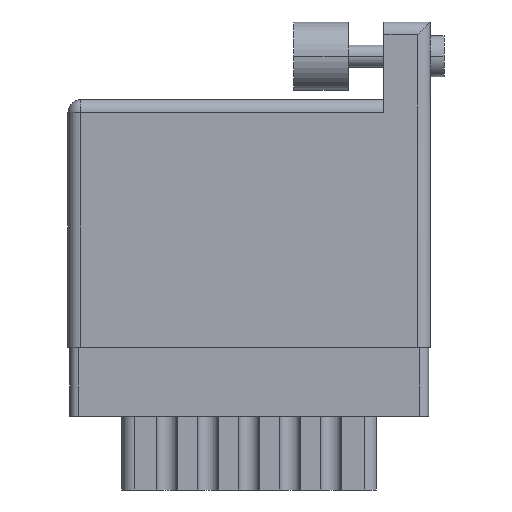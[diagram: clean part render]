
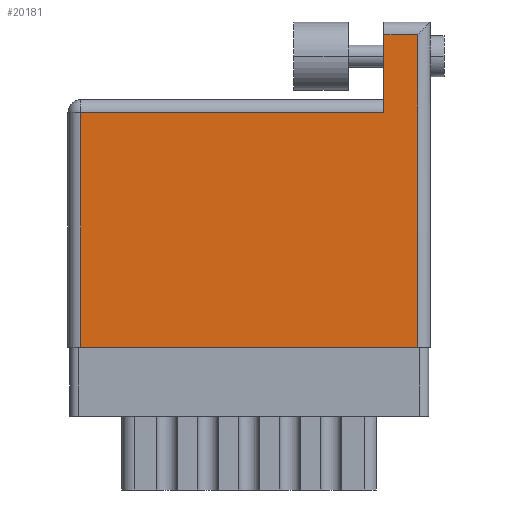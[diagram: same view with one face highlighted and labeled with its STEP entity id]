
A CAD part, front view. The second image highlights one B-rep face of the part: STEP entity #20181.
In plain terms, the highlighted face is planar.
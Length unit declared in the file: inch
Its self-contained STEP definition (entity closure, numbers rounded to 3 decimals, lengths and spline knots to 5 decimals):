
#1855 = CARTESIAN_POINT ( 'NONE',  ( 0., 0.859, 0. ) ) ;
#1906 = DIRECTION ( 'NONE',  ( 0., 1., 0. ) ) ;
#3386 = CARTESIAN_POINT ( 'NONE',  ( 1.155, 1.19, 0. ) ) ;
#3553 = VERTEX_POINT ( 'NONE', #25273 ) ;
#4104 = VERTEX_POINT ( 'NONE', #6289 ) ;
#4347 = LINE ( 'NONE', #1855, #9684 ) ;
#4431 = EDGE_CURVE ( 'NONE', #9054, #4104, #13331, .T. ) ;
#5066 = EDGE_CURVE ( 'NONE', #5283, #9054, #16066, .T. ) ;
#5283 = VERTEX_POINT ( 'NONE', #16950 ) ;
#5483 = LINE ( 'NONE', #3386, #15075 ) ;
#6289 = CARTESIAN_POINT ( 'NONE',  ( 1.155, 1.143, 0. ) ) ;
#7041 = VERTEX_POINT ( 'NONE', #9568 ) ;
#7189 = DIRECTION ( 'NONE',  ( -1., 0., 0. ) ) ;
#7658 = VECTOR ( 'NONE', #8145, 39.37008 ) ;
#7846 = ORIENTED_EDGE ( 'NONE', *, *, #21690, .T. ) ;
#7950 = CARTESIAN_POINT ( 'NONE',  ( 1.278, 1.143, 0. ) ) ;
#8145 = DIRECTION ( 'NONE',  ( 1., 0., 0. ) ) ;
#9054 = VERTEX_POINT ( 'NONE', #7950 ) ;
#9568 = CARTESIAN_POINT ( 'NONE',  ( 0.047, 0., 0. ) ) ;
#9684 = VECTOR ( 'NONE', #23977, 39.37008 ) ;
#9896 = CARTESIAN_POINT ( 'NONE',  ( 1.278, 1.19, 0. ) ) ;
#10797 = CARTESIAN_POINT ( 'NONE',  ( 0.047, 0.859, 0. ) ) ;
#11574 = LINE ( 'NONE', #21392, #7658 ) ;
#12564 = VECTOR ( 'NONE', #1906, 39.37008 ) ;
#13205 = DIRECTION ( 'NONE',  ( 0., -1., 0. ) ) ;
#13311 = DIRECTION ( 'NONE',  ( 0., 0., -1. ) ) ;
#13331 = LINE ( 'NONE', #23404, #21728 ) ;
#13974 = EDGE_LOOP ( 'NONE', ( #7846, #18714, #19465, #24093, #22214, #21532 ) ) ;
#14175 = EDGE_CURVE ( 'NONE', #4104, #3553, #5483, .T. ) ;
#15075 = VECTOR ( 'NONE', #13205, 39.37008 ) ;
#15550 = CARTESIAN_POINT ( 'NONE',  ( 0., 0.906, 0. ) ) ;
#16014 = EDGE_CURVE ( 'NONE', #22884, #7041, #19489, .T. ) ;
#16066 = LINE ( 'NONE', #9896, #12564 ) ;
#16950 = CARTESIAN_POINT ( 'NONE',  ( 1.278, 0., 0. ) ) ;
#17516 = DIRECTION ( 'NONE',  ( 0., -1., 0. ) ) ;
#17633 = AXIS2_PLACEMENT_3D ( 'NONE', #15550, #13311, #23523 ) ;
#18714 = ORIENTED_EDGE ( 'NONE', *, *, #5066, .T. ) ;
#19077 = PLANE ( 'NONE',  #17633 ) ;
#19465 = ORIENTED_EDGE ( 'NONE', *, *, #4431, .T. ) ;
#19489 = LINE ( 'NONE', #25244, #24119 ) ;
#20181 = ADVANCED_FACE ( 'NONE', ( #25229 ), #19077, .F. ) ;
#21392 = CARTESIAN_POINT ( 'NONE',  ( 0., 0., 0. ) ) ;
#21532 = ORIENTED_EDGE ( 'NONE', *, *, #16014, .T. ) ;
#21690 = EDGE_CURVE ( 'NONE', #7041, #5283, #11574, .T. ) ;
#21728 = VECTOR ( 'NONE', #7189, 39.37008 ) ;
#22214 = ORIENTED_EDGE ( 'NONE', *, *, #23733, .T. ) ;
#22884 = VERTEX_POINT ( 'NONE', #10797 ) ;
#23404 = CARTESIAN_POINT ( 'NONE',  ( 1.155, 1.143, 0. ) ) ;
#23523 = DIRECTION ( 'NONE',  ( -1., 0., 0. ) ) ;
#23733 = EDGE_CURVE ( 'NONE', #3553, #22884, #4347, .T. ) ;
#23977 = DIRECTION ( 'NONE',  ( -1., 0., 0. ) ) ;
#24093 = ORIENTED_EDGE ( 'NONE', *, *, #14175, .T. ) ;
#24119 = VECTOR ( 'NONE', #17516, 39.37008 ) ;
#25229 = FACE_OUTER_BOUND ( 'NONE', #13974, .T. ) ;
#25244 = CARTESIAN_POINT ( 'NONE',  ( 0.047, 0., 0. ) ) ;
#25273 = CARTESIAN_POINT ( 'NONE',  ( 1.155, 0.859, 0. ) ) ;
